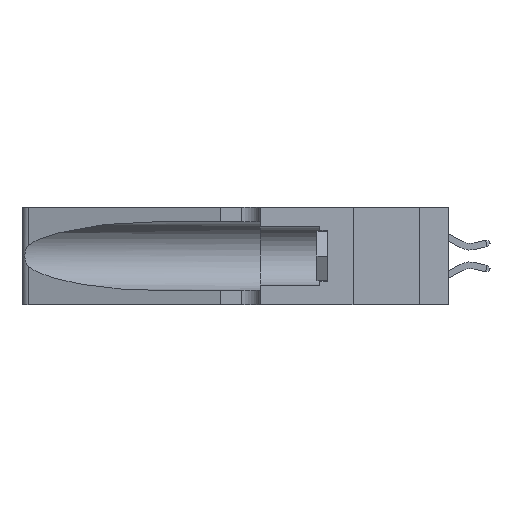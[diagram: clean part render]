
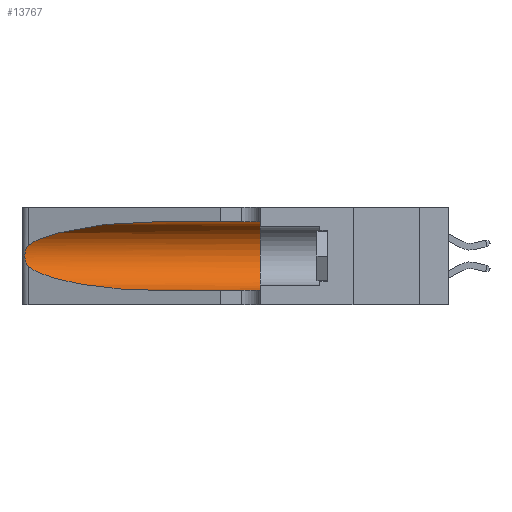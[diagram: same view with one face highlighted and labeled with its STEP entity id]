
A CAD part, left-side view. The second image highlights one B-rep face of the part: STEP entity #13767.
In plain terms, the highlighted cylindrical face has radius 3.308 mm (diameter 6.617 mm), a partial arc.
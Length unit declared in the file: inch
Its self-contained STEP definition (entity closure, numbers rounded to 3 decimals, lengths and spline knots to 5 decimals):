
#78 = FACE_OUTER_BOUND ( 'NONE', #1924, .T. ) ;
#807 = CARTESIAN_POINT ( 'NONE',  ( 0.26018, 1.23835, 0.19895 ) ) ;
#1002 = VERTEX_POINT ( 'NONE', #10946 ) ;
#1175 = CARTESIAN_POINT ( 'NONE',  ( 0.1305, 1.61858, 0.185 ) ) ;
#1415 = EDGE_CURVE ( 'NONE', #19614, #7073, #12692, .T. ) ;
#1527 = ORIENTED_EDGE ( 'NONE', *, *, #27915, .T. ) ;
#1924 = EDGE_LOOP ( 'NONE', ( #14287, #1527, #2178, #2950, #8630, #5499 ) ) ;
#1989 = CARTESIAN_POINT ( 'NONE',  ( 0.1305, 0.72297, 0.31525 ) ) ;
#2178 = ORIENTED_EDGE ( 'NONE', *, *, #10460, .T. ) ;
#2950 = ORIENTED_EDGE ( 'NONE', *, *, #19594, .T. ) ;
#3416 = CARTESIAN_POINT ( 'NONE',  ( 0.26075, 1.23896, 0.178 ) ) ;
#4618 = CARTESIAN_POINT ( 'NONE',  ( 0.25487, 1.22718, 0.22369 ) ) ;
#5499 = ORIENTED_EDGE ( 'NONE', *, *, #14427, .F. ) ;
#6035 = CARTESIAN_POINT ( 'NONE',  ( 0.2373, 1.15595, 0.08982 ) ) ;
#6088 = CARTESIAN_POINT ( 'NONE',  ( 0.25856, 1.23593, 0.16098 ) ) ;
#7073 = VERTEX_POINT ( 'NONE', #7331 ) ;
#7331 = CARTESIAN_POINT ( 'NONE',  ( 0.1305, 0.35, 0.05475 ) ) ;
#8630 = ORIENTED_EDGE ( 'NONE', *, *, #1415, .F. ) ;
#8712 = CARTESIAN_POINT ( 'NONE',  ( 0.25639, 1.23186, 0.15144 ) ) ;
#9482 = CARTESIAN_POINT ( 'NONE',  ( 0.1305, 0.35, 0.185 ) ) ;
#9636 = DIRECTION ( 'NONE',  ( 0., 1., 0. ) ) ;
#9700 = DIRECTION ( 'NONE',  ( 0., 0., 1. ) ) ;
#9885 = B_SPLINE_CURVE_WITH_KNOTS ( 'NONE', 3,
 ( #11213, #23805, #13790, #31265, #16320, #807, #18926, #3416, #21438, #6088, #23908, #8712, #26425, #11321 ),
 .UNSPECIFIED., .F., .F.,
 ( 4, 2, 2, 2, 2, 2, 4 ),
 ( 0., 0.00027, 0.00053, 0.00107, 0.0016, 0.00187, 0.00214 ),
 .UNSPECIFIED. ) ;
#10273 = CARTESIAN_POINT ( 'NONE',  ( 0.1305, 0.72297, 0.31525 ) ) ;
#10460 = EDGE_CURVE ( 'NONE', #28136, #11573, #14797, .T. ) ;
#10946 = CARTESIAN_POINT ( 'NONE',  ( 0.25487, 1.22718, 0.22369 ) ) ;
#11076 = AXIS2_PLACEMENT_3D ( 'NONE', #9482, #9636, #9700 ) ;
#11213 = CARTESIAN_POINT ( 'NONE',  ( 0.25487, 1.22718, 0.22369 ) ) ;
#11321 = CARTESIAN_POINT ( 'NONE',  ( 0.25487, 1.22718, 0.14631 ) ) ;
#11573 = VERTEX_POINT ( 'NONE', #30623 ) ;
#11769 = CARTESIAN_POINT ( 'NONE',  ( 0.1305, 0.35, 0.31525 ) ) ;
#12692 = CIRCLE ( 'NONE', #11076, 0.13025 ) ;
#13767 = ADVANCED_FACE ( 'NONE', ( #78 ), #31514, .F. ) ;
#13790 = CARTESIAN_POINT ( 'NONE',  ( 0.25639, 1.23184, 0.21858 ) ) ;
#13851 = CARTESIAN_POINT ( 'NONE',  ( 0.25487, 1.22718, 0.14631 ) ) ;
#14287 = ORIENTED_EDGE ( 'NONE', *, *, #16215, .T. ) ;
#14306 = CARTESIAN_POINT ( 'NONE',  ( 0.1305, 1.61858, 0.05475 ) ) ;
#14427 = EDGE_CURVE ( 'NONE', #17718, #19614, #26080, .T. ) ;
#14797 =( BOUNDED_CURVE ( )  B_SPLINE_CURVE ( 3, ( #13851, #6035, #16273, #31329 ),
 .UNSPECIFIED., .F., .T. ) 
 B_SPLINE_CURVE_WITH_KNOTS ( ( 4, 4 ),
 ( 3.44316, 4.71239 ),
 .UNSPECIFIED. ) 
 CURVE ( )  GEOMETRIC_REPRESENTATION_ITEM ( )  RATIONAL_B_SPLINE_CURVE ( ( 1., 0.87, 0.87, 1. ) ) 
 REPRESENTATION_ITEM ( '' )  );
#16215 = EDGE_CURVE ( 'NONE', #17718, #1002, #24071, .T. ) ;
#16273 = CARTESIAN_POINT ( 'NONE',  ( 0.18966, 0.96281, 0.05475 ) ) ;
#16320 = CARTESIAN_POINT ( 'NONE',  ( 0.25854, 1.2359, 0.20912 ) ) ;
#16521 = DIRECTION ( 'NONE',  ( 0., -1., 0. ) ) ;
#16670 = DIRECTION ( 'NONE',  ( 0., -1., 0. ) ) ;
#16873 = DIRECTION ( 'NONE',  ( 0., -1., 0. ) ) ;
#17340 = CARTESIAN_POINT ( 'NONE',  ( 0.25487, 1.22718, 0.14631 ) ) ;
#17519 = CARTESIAN_POINT ( 'NONE',  ( 0.18966, 0.96281, 0.31525 ) ) ;
#17718 = VERTEX_POINT ( 'NONE', #10273 ) ;
#18926 = CARTESIAN_POINT ( 'NONE',  ( 0.26075, 1.23896, 0.19203 ) ) ;
#19471 = VECTOR ( 'NONE', #16521, 39.37008 ) ;
#19594 = EDGE_CURVE ( 'NONE', #11573, #7073, #20372, .T. ) ;
#19614 = VERTEX_POINT ( 'NONE', #11769 ) ;
#19847 = AXIS2_PLACEMENT_3D ( 'NONE', #1175, #16670, #24130 ) ;
#20073 = CARTESIAN_POINT ( 'NONE',  ( 0.2373, 1.15595, 0.28018 ) ) ;
#20372 = LINE ( 'NONE', #14306, #32728 ) ;
#21438 = CARTESIAN_POINT ( 'NONE',  ( 0.26017, 1.23833, 0.17102 ) ) ;
#23805 = CARTESIAN_POINT ( 'NONE',  ( 0.25555, 1.22994, 0.2215 ) ) ;
#23908 = CARTESIAN_POINT ( 'NONE',  ( 0.25789, 1.23486, 0.15765 ) ) ;
#24071 =( BOUNDED_CURVE ( )  B_SPLINE_CURVE ( 3, ( #1989, #17519, #20073, #4618 ),
 .UNSPECIFIED., .F., .F. ) 
 B_SPLINE_CURVE_WITH_KNOTS ( ( 4, 4 ),
 ( 1.5708, 2.84003 ),
 .UNSPECIFIED. ) 
 CURVE ( )  GEOMETRIC_REPRESENTATION_ITEM ( )  RATIONAL_B_SPLINE_CURVE ( ( 1., 0.87, 0.87, 1. ) ) 
 REPRESENTATION_ITEM ( '' )  );
#24130 = DIRECTION ( 'NONE',  ( 0., 0., -1. ) ) ;
#26080 = LINE ( 'NONE', #28987, #19471 ) ;
#26425 = CARTESIAN_POINT ( 'NONE',  ( 0.25555, 1.22993, 0.14849 ) ) ;
#27915 = EDGE_CURVE ( 'NONE', #1002, #28136, #9885, .T. ) ;
#28136 = VERTEX_POINT ( 'NONE', #17340 ) ;
#28987 = CARTESIAN_POINT ( 'NONE',  ( 0.1305, 1.61858, 0.31525 ) ) ;
#30623 = CARTESIAN_POINT ( 'NONE',  ( 0.1305, 0.72297, 0.05475 ) ) ;
#31265 = CARTESIAN_POINT ( 'NONE',  ( 0.25787, 1.23484, 0.2124 ) ) ;
#31329 = CARTESIAN_POINT ( 'NONE',  ( 0.1305, 0.72297, 0.05475 ) ) ;
#31514 = CYLINDRICAL_SURFACE ( 'NONE', #19847, 0.13025 ) ;
#32728 = VECTOR ( 'NONE', #16873, 39.37008 ) ;
